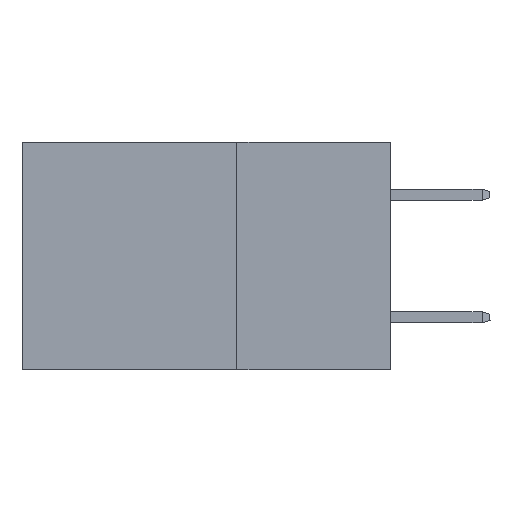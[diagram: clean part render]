
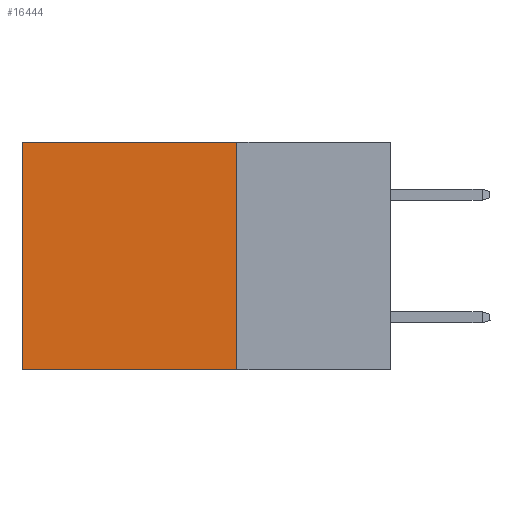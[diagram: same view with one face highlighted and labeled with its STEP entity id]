
A CAD part, left-side view. The second image highlights one B-rep face of the part: STEP entity #16444.
In plain terms, the highlighted planar face has unit normal (-1, 0, 0).
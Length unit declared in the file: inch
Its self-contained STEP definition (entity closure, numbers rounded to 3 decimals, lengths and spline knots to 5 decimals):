
#676 = CARTESIAN_POINT ( 'NONE',  ( 0.2875, 0.25, 0. ) ) ;
#1079 = DIRECTION ( 'NONE',  ( 0., 0., -1. ) ) ;
#2238 = VERTEX_POINT ( 'NONE', #3062 ) ;
#2528 = EDGE_CURVE ( 'NONE', #2238, #19902, #14736, .T. ) ;
#3062 = CARTESIAN_POINT ( 'NONE',  ( 0.2875, 0.25, 0. ) ) ;
#3370 = LINE ( 'NONE', #676, #32384 ) ;
#4304 = CARTESIAN_POINT ( 'NONE',  ( 0.2875, 0.6, 0. ) ) ;
#5398 = VERTEX_POINT ( 'NONE', #7401 ) ;
#5579 = DIRECTION ( 'NONE',  ( 1., 0., 0. ) ) ;
#6455 = ORIENTED_EDGE ( 'NONE', *, *, #21536, .T. ) ;
#6546 = EDGE_CURVE ( 'NONE', #2238, #30329, #3370, .T. ) ;
#7401 = CARTESIAN_POINT ( 'NONE',  ( 0.2875, 0.6, -0.37 ) ) ;
#8222 = DIRECTION ( 'NONE',  ( 0., 1., 0. ) ) ;
#9455 = CARTESIAN_POINT ( 'NONE',  ( 0.2875, 0.25, -0.37 ) ) ;
#9816 = AXIS2_PLACEMENT_3D ( 'NONE', #30138, #5579, #32107 ) ;
#10148 = VECTOR ( 'NONE', #26635, 39.37008 ) ;
#12369 = ORIENTED_EDGE ( 'NONE', *, *, #2528, .F. ) ;
#14736 = LINE ( 'NONE', #25649, #30442 ) ;
#15636 = ORIENTED_EDGE ( 'NONE', *, *, #6546, .T. ) ;
#16074 = CARTESIAN_POINT ( 'NONE',  ( 0.2875, 0.25, -0.37 ) ) ;
#16432 = ORIENTED_EDGE ( 'NONE', *, *, #24726, .F. ) ;
#16444 = ADVANCED_FACE ( 'NONE', ( #21208 ), #32818, .F. ) ;
#17170 = CARTESIAN_POINT ( 'NONE',  ( 0.2875, 0.6, 0. ) ) ;
#19902 = VERTEX_POINT ( 'NONE', #9455 ) ;
#21208 = FACE_OUTER_BOUND ( 'NONE', #21659, .T. ) ;
#21536 = EDGE_CURVE ( 'NONE', #30329, #5398, #25917, .T. ) ;
#21642 = LINE ( 'NONE', #16074, #10148 ) ;
#21659 = EDGE_LOOP ( 'NONE', ( #6455, #16432, #12369, #15636 ) ) ;
#24726 = EDGE_CURVE ( 'NONE', #19902, #5398, #21642, .T. ) ;
#25649 = CARTESIAN_POINT ( 'NONE',  ( 0.2875, 0.25, 0. ) ) ;
#25917 = LINE ( 'NONE', #17170, #34625 ) ;
#26635 = DIRECTION ( 'NONE',  ( 0., 1., 0. ) ) ;
#30138 = CARTESIAN_POINT ( 'NONE',  ( 0.2875, 0.25, 0. ) ) ;
#30329 = VERTEX_POINT ( 'NONE', #4304 ) ;
#30442 = VECTOR ( 'NONE', #1079, 39.37008 ) ;
#31466 = DIRECTION ( 'NONE',  ( 0., 0., -1. ) ) ;
#32107 = DIRECTION ( 'NONE',  ( 0., 0., -1. ) ) ;
#32384 = VECTOR ( 'NONE', #8222, 39.37008 ) ;
#32818 = PLANE ( 'NONE',  #9816 ) ;
#34625 = VECTOR ( 'NONE', #31466, 39.37008 ) ;
